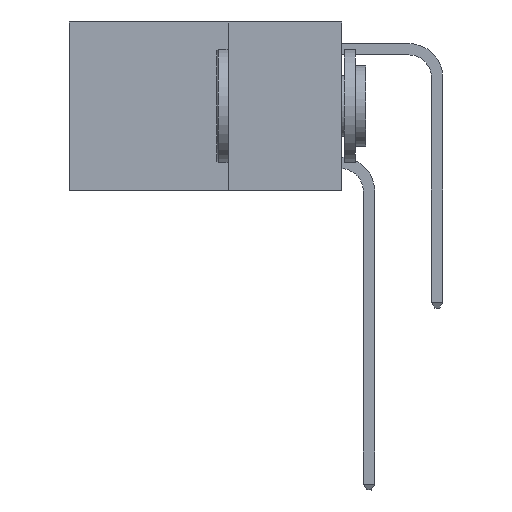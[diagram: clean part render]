
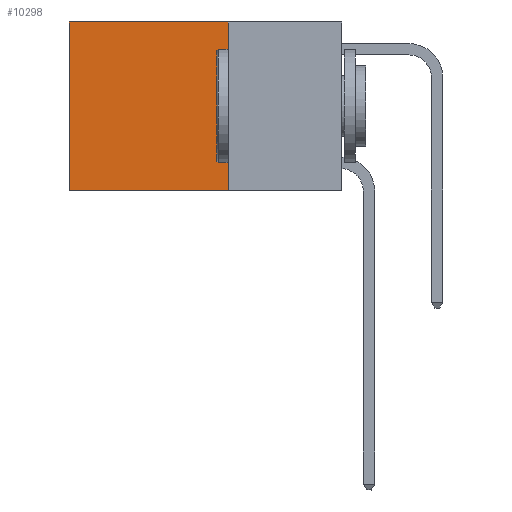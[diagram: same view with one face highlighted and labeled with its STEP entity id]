
A CAD part, left-side view. The second image highlights one B-rep face of the part: STEP entity #10298.
In plain terms, the highlighted planar face has unit normal (-1, 0, 0).
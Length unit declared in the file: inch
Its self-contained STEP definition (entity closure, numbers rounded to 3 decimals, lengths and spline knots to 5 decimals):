
#170 = ORIENTED_EDGE ( 'NONE', *, *, #17449, .F. ) ;
#933 = VECTOR ( 'NONE', #20498, 39.37008 ) ;
#1804 = EDGE_CURVE ( 'NONE', #7009, #22273, #16280, .T. ) ;
#3287 = CARTESIAN_POINT ( 'NONE',  ( 0.2625, 0.25, 0. ) ) ;
#4626 = AXIS2_PLACEMENT_3D ( 'NONE', #7105, #18590, #7188 ) ;
#5051 = FACE_OUTER_BOUND ( 'NONE', #14063, .T. ) ;
#5073 = DIRECTION ( 'NONE',  ( 0., 1., 0. ) ) ;
#5550 = CARTESIAN_POINT ( 'NONE',  ( 0.2625, 0.25, -0.37 ) ) ;
#6124 = CARTESIAN_POINT ( 'NONE',  ( 0.2625, 0.25, 0. ) ) ;
#6139 = VECTOR ( 'NONE', #5073, 39.37008 ) ;
#7009 = VERTEX_POINT ( 'NONE', #20362 ) ;
#7105 = CARTESIAN_POINT ( 'NONE',  ( 0.2625, 0.25, 0. ) ) ;
#7188 = DIRECTION ( 'NONE',  ( 0., 0., -1. ) ) ;
#7549 = CARTESIAN_POINT ( 'NONE',  ( 0.2625, 0.6, 0. ) ) ;
#8079 = EDGE_CURVE ( 'NONE', #20453, #13693, #9075, .T. ) ;
#8986 = PLANE ( 'NONE',  #4626 ) ;
#9075 = LINE ( 'NONE', #13814, #18640 ) ;
#10298 = ADVANCED_FACE ( 'NONE', ( #5051 ), #8986, .F. ) ;
#11344 = VECTOR ( 'NONE', #20821, 39.37008 ) ;
#12650 = ORIENTED_EDGE ( 'NONE', *, *, #8079, .T. ) ;
#13693 = VERTEX_POINT ( 'NONE', #19379 ) ;
#13814 = CARTESIAN_POINT ( 'NONE',  ( 0.2625, 0.25, 0. ) ) ;
#14063 = EDGE_LOOP ( 'NONE', ( #17664, #20834, #170, #12650 ) ) ;
#14173 = EDGE_CURVE ( 'NONE', #13693, #22273, #20276, .T. ) ;
#16280 = LINE ( 'NONE', #5550, #6139 ) ;
#17140 = CARTESIAN_POINT ( 'NONE',  ( 0.2625, 0.6, -0.37 ) ) ;
#17449 = EDGE_CURVE ( 'NONE', #20453, #7009, #20706, .T. ) ;
#17664 = ORIENTED_EDGE ( 'NONE', *, *, #14173, .T. ) ;
#17692 = DIRECTION ( 'NONE',  ( 0., 1., 0. ) ) ;
#18590 = DIRECTION ( 'NONE',  ( 1., 0., 0. ) ) ;
#18640 = VECTOR ( 'NONE', #17692, 39.37008 ) ;
#19379 = CARTESIAN_POINT ( 'NONE',  ( 0.2625, 0.6, 0. ) ) ;
#20276 = LINE ( 'NONE', #7549, #11344 ) ;
#20362 = CARTESIAN_POINT ( 'NONE',  ( 0.2625, 0.25, -0.37 ) ) ;
#20453 = VERTEX_POINT ( 'NONE', #6124 ) ;
#20498 = DIRECTION ( 'NONE',  ( 0., 0., -1. ) ) ;
#20706 = LINE ( 'NONE', #3287, #933 ) ;
#20821 = DIRECTION ( 'NONE',  ( 0., 0., -1. ) ) ;
#20834 = ORIENTED_EDGE ( 'NONE', *, *, #1804, .F. ) ;
#22273 = VERTEX_POINT ( 'NONE', #17140 ) ;
